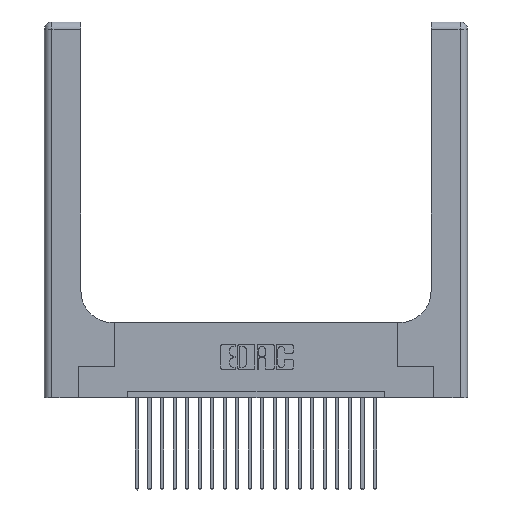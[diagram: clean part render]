
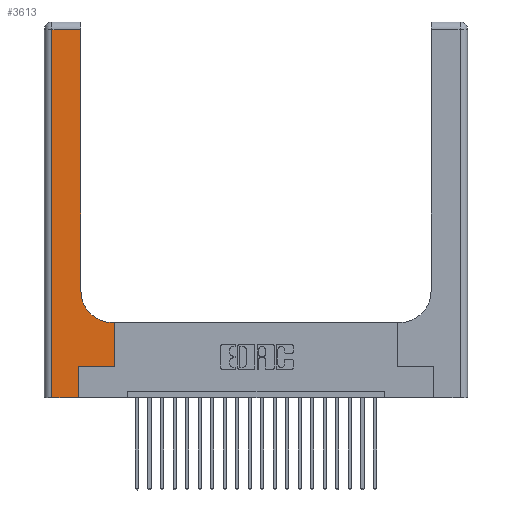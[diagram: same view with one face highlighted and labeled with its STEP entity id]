
A CAD part, top view. The second image highlights one B-rep face of the part: STEP entity #3613.
In plain terms, the highlighted planar face has unit normal (0, 0, 1).
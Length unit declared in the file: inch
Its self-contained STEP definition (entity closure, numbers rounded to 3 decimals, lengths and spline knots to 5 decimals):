
#52 = VERTEX_POINT ( 'NONE', #3130 ) ;
#1192 = CARTESIAN_POINT ( 'NONE',  ( 0.5415, 0.6, 0.37 ) ) ;
#1277 = CARTESIAN_POINT ( 'NONE',  ( 0.5415, 0.85, 0.37 ) ) ;
#1426 = DIRECTION ( 'NONE',  ( 0., 1., 0. ) ) ;
#1636 = VERTEX_POINT ( 'NONE', #13160 ) ;
#1723 = EDGE_LOOP ( 'NONE', ( #19440, #6457, #2082, #13735, #17139, #8067, #8970, #2885, #9280 ) ) ;
#2082 = ORIENTED_EDGE ( 'NONE', *, *, #22501, .T. ) ;
#2158 = VERTEX_POINT ( 'NONE', #7223 ) ;
#2885 = ORIENTED_EDGE ( 'NONE', *, *, #21719, .T. ) ;
#3127 = VERTEX_POINT ( 'NONE', #19137 ) ;
#3130 = CARTESIAN_POINT ( 'NONE',  ( 0.5585, 0.25, 0.37 ) ) ;
#3432 = LINE ( 'NONE', #4614, #21383 ) ;
#3484 = EDGE_CURVE ( 'NONE', #9797, #2158, #4660, .T. ) ;
#3613 = ADVANCED_FACE ( 'NONE', ( #14766 ), #9936, .F. ) ;
#3890 = LINE ( 'NONE', #22757, #8419 ) ;
#4614 = CARTESIAN_POINT ( 'NONE',  ( 0.06, 3., 0.37 ) ) ;
#4660 = CIRCLE ( 'NONE', #15634, 0.25 ) ;
#5355 = VERTEX_POINT ( 'NONE', #21381 ) ;
#5427 = VERTEX_POINT ( 'NONE', #12985 ) ;
#5830 = VECTOR ( 'NONE', #21890, 39.37008 ) ;
#6457 = ORIENTED_EDGE ( 'NONE', *, *, #20931, .T. ) ;
#7223 = CARTESIAN_POINT ( 'NONE',  ( 0.2915, 0.85, 0.37 ) ) ;
#7831 = CARTESIAN_POINT ( 'NONE',  ( 0.06, 2.94, 0.37 ) ) ;
#8067 = ORIENTED_EDGE ( 'NONE', *, *, #14829, .T. ) ;
#8223 = DIRECTION ( 'NONE',  ( 0., 0., -1. ) ) ;
#8419 = VECTOR ( 'NONE', #13665, 39.37008 ) ;
#8648 = CARTESIAN_POINT ( 'NONE',  ( 0.5585, 0.25, 0.37 ) ) ;
#8721 = DIRECTION ( 'NONE',  ( 0., 1., 0. ) ) ;
#8970 = ORIENTED_EDGE ( 'NONE', *, *, #10928, .T. ) ;
#9280 = ORIENTED_EDGE ( 'NONE', *, *, #3484, .T. ) ;
#9284 = DIRECTION ( 'NONE',  ( 1., 0., 0. ) ) ;
#9376 = CARTESIAN_POINT ( 'NONE',  ( 0.269, 0.25, 0.37 ) ) ;
#9620 = AXIS2_PLACEMENT_3D ( 'NONE', #22407, #8223, #20759 ) ;
#9797 = VERTEX_POINT ( 'NONE', #1192 ) ;
#9875 = DIRECTION ( 'NONE',  ( 0., -1., 0. ) ) ;
#9936 = PLANE ( 'NONE',  #9620 ) ;
#10928 = EDGE_CURVE ( 'NONE', #52, #5427, #17146, .T. ) ;
#11039 = EDGE_CURVE ( 'NONE', #2158, #1636, #14045, .T. ) ;
#11556 = LINE ( 'NONE', #14034, #22226 ) ;
#11811 = VECTOR ( 'NONE', #1426, 39.37008 ) ;
#11972 = EDGE_CURVE ( 'NONE', #20789, #3127, #16534, .T. ) ;
#12505 = DIRECTION ( 'NONE',  ( 0., 0., -1. ) ) ;
#12985 = CARTESIAN_POINT ( 'NONE',  ( 0.5585, 0.6, 0.37 ) ) ;
#13160 = CARTESIAN_POINT ( 'NONE',  ( 0.2915, 2.94, 0.37 ) ) ;
#13442 = CARTESIAN_POINT ( 'NONE',  ( 0., 0., 0.37 ) ) ;
#13588 = LINE ( 'NONE', #9376, #18942 ) ;
#13665 = DIRECTION ( 'NONE',  ( -1., 0., 0. ) ) ;
#13735 = ORIENTED_EDGE ( 'NONE', *, *, #11972, .T. ) ;
#14034 = CARTESIAN_POINT ( 'NONE',  ( 0.269, 0., 0.37 ) ) ;
#14045 = LINE ( 'NONE', #14507, #23012 ) ;
#14507 = CARTESIAN_POINT ( 'NONE',  ( 0.2915, 3., 0.37 ) ) ;
#14766 = FACE_OUTER_BOUND ( 'NONE', #1723, .T. ) ;
#14829 = EDGE_CURVE ( 'NONE', #5355, #52, #13588, .T. ) ;
#15253 = CARTESIAN_POINT ( 'NONE',  ( 0.06, 0., 0.37 ) ) ;
#15576 = DIRECTION ( 'NONE',  ( 1., 0., 0. ) ) ;
#15634 = AXIS2_PLACEMENT_3D ( 'NONE', #1277, #12505, #15654 ) ;
#15654 = DIRECTION ( 'NONE',  ( 1., 0., 0. ) ) ;
#16246 = VECTOR ( 'NONE', #15576, 39.37008 ) ;
#16396 = DIRECTION ( 'NONE',  ( 0., 1., 0. ) ) ;
#16492 = CARTESIAN_POINT ( 'NONE',  ( 0.2915, 0.6, 0.37 ) ) ;
#16534 = LINE ( 'NONE', #13442, #16246 ) ;
#16772 = LINE ( 'NONE', #16492, #5830 ) ;
#17139 = ORIENTED_EDGE ( 'NONE', *, *, #21984, .T. ) ;
#17146 = LINE ( 'NONE', #8648, #11811 ) ;
#18942 = VECTOR ( 'NONE', #9284, 39.37008 ) ;
#19137 = CARTESIAN_POINT ( 'NONE',  ( 0.269, 0., 0.37 ) ) ;
#19440 = ORIENTED_EDGE ( 'NONE', *, *, #11039, .T. ) ;
#20759 = DIRECTION ( 'NONE',  ( -1., 0., 0. ) ) ;
#20789 = VERTEX_POINT ( 'NONE', #15253 ) ;
#20931 = EDGE_CURVE ( 'NONE', #1636, #22304, #3890, .T. ) ;
#21381 = CARTESIAN_POINT ( 'NONE',  ( 0.269, 0.25, 0.37 ) ) ;
#21383 = VECTOR ( 'NONE', #9875, 39.37008 ) ;
#21719 = EDGE_CURVE ( 'NONE', #5427, #9797, #16772, .T. ) ;
#21890 = DIRECTION ( 'NONE',  ( -1., 0., 0. ) ) ;
#21984 = EDGE_CURVE ( 'NONE', #3127, #5355, #11556, .T. ) ;
#22226 = VECTOR ( 'NONE', #8721, 39.37008 ) ;
#22304 = VERTEX_POINT ( 'NONE', #7831 ) ;
#22407 = CARTESIAN_POINT ( 'NONE',  ( 0., 3., 0.37 ) ) ;
#22501 = EDGE_CURVE ( 'NONE', #22304, #20789, #3432, .T. ) ;
#22757 = CARTESIAN_POINT ( 'NONE',  ( 0., 2.94, 0.37 ) ) ;
#23012 = VECTOR ( 'NONE', #16396, 39.37008 ) ;
